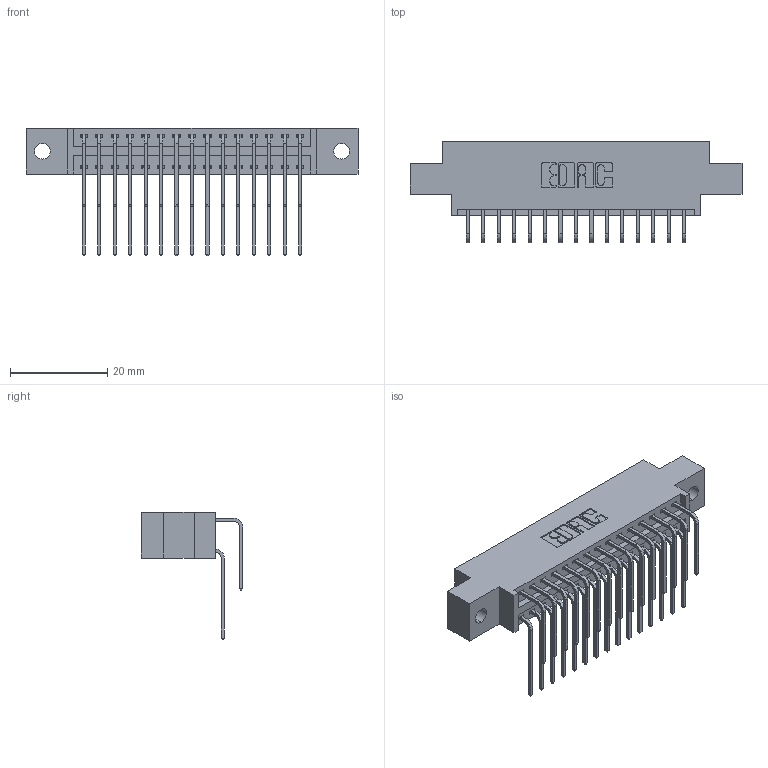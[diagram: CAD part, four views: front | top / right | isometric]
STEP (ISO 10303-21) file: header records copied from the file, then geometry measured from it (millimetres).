
FILE_DESCRIPTION (( 'STEP AP203' ), '1' );
FILE_NAME ('396-030-559-802.STEP', '2018-09-05T08:13:22', ( '' ), ( '' ), 'SwSTEP 2.0', 'SolidWorks 2016', '' );
FILE_SCHEMA (( 'CONFIG_CONTROL_DESIGN' ));
Length unit declared in the file: inch
Products named in the file (4): 346 Part_0.170 Offset - 0.128 Dia; 345-292-001_558 559 Tail - 1; 345-292-001_559 Tail - 2; 396-030-559-802
Assembly tree (31 placements, depth 2):
  396-030-559-802
    346 Part_0.170 Offset - 0.128 Dia
    345-292-001_558 559 Tail - 1  x15
    345-292-001_559 Tail - 2  x15
Bounding box: 68.2 x 20.89 x 26.16 mm (x, y, z)
Volume: 6422.3 mm3; surface area: 9144.1 mm2
Topology: 31 solids, 31 shells, 1746 faces, 5171 edges, 3406 vertices
Faces by surface type: plane 1190, cylinder 556
Entity records: 15343 total; most frequent: CARTESIAN_POINT 2619, ORIENTED_EDGE 2502, DIRECTION 2331, EDGE_CURVE 1251, LINE 1019, VECTOR 1019, VERTEX_POINT 830, AXIS2_PLACEMENT_3D 656
